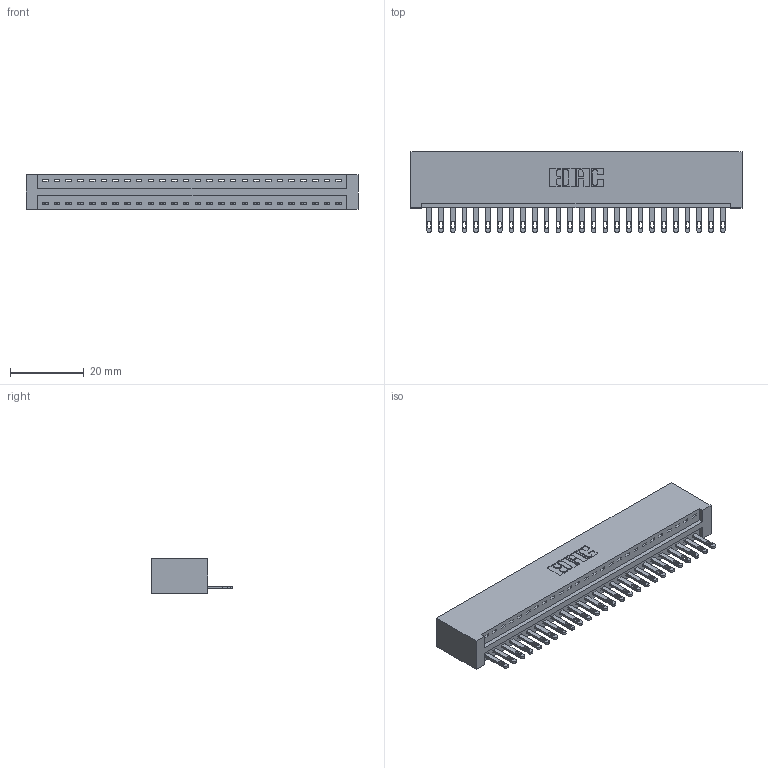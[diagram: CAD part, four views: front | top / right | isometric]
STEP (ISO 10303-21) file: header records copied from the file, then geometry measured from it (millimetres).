
FILE_DESCRIPTION (( 'STEP AP203' ), '1' );
FILE_NAME ('896-026-500-101.STEP', '2021-07-27T17:46:07', ( '' ), ( '' ), 'SwSTEP 2.0', 'SolidWorks 2020', '' );
FILE_SCHEMA (( 'CONFIG_CONTROL_DESIGN' ));
Length unit declared in the file: inch
Products named in the file (3): 345-292-001_345-293-100; 846 Part_No Mounting Lugs; 896-026-500-101
Assembly tree (27 placements, depth 2):
  896-026-500-101
    846 Part_No Mounting Lugs
    345-292-001_345-293-100  x26
Bounding box: 89.79 x 21.84 x 9.4 mm (x, y, z)
Volume: 9050.1 mm3; surface area: 11274.4 mm2
Topology: 27 solids, 27 shells, 1518 faces, 4673 edges, 3114 vertices
Faces by surface type: plane 956, cylinder 562
Entity records: 17943 total; most frequent: CARTESIAN_POINT 3086, ORIENTED_EDGE 3046, DIRECTION 2739, EDGE_CURVE 1523, LINE 1291, VECTOR 1291, VERTEX_POINT 1014, AXIS2_PLACEMENT_3D 724
